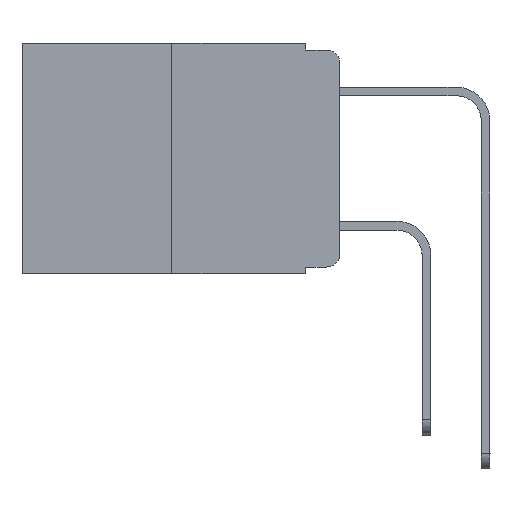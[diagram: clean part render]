
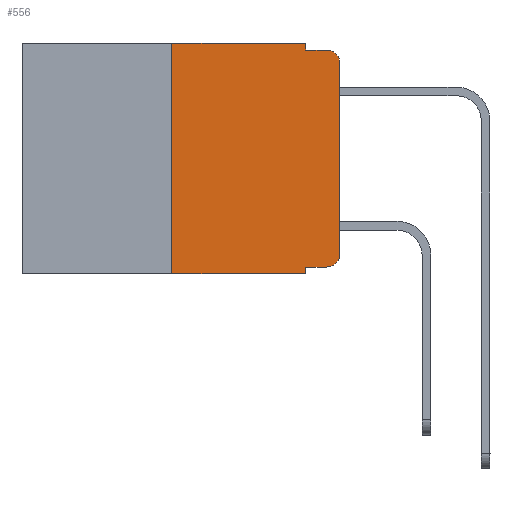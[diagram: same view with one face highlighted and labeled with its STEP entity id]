
A CAD part, left-side view. The second image highlights one B-rep face of the part: STEP entity #556.
In plain terms, the highlighted planar face has unit normal (-1, 0, 0).
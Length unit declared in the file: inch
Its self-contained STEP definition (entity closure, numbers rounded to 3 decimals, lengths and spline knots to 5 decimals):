
#143 = VERTEX_POINT ( 'NONE', #16072 ) ;
#154 = CARTESIAN_POINT ( 'NONE',  ( 0., 0.051, 0. ) ) ;
#478 = EDGE_CURVE ( 'NONE', #11710, #15824, #767, .T. ) ;
#556 = ADVANCED_FACE ( 'NONE', ( #12794 ), #1880, .F. ) ;
#623 = CIRCLE ( 'NONE', #14624, 0.02 ) ;
#665 = AXIS2_PLACEMENT_3D ( 'NONE', #14664, #6798, #13257 ) ;
#767 = LINE ( 'NONE', #4546, #13063 ) ;
#1188 = CARTESIAN_POINT ( 'NONE',  ( 0., 0.051, 0. ) ) ;
#1325 = CARTESIAN_POINT ( 'NONE',  ( 0., 0.051, 0. ) ) ;
#1472 = VERTEX_POINT ( 'NONE', #18660 ) ;
#1818 = DIRECTION ( 'NONE',  ( -1., 0., 0. ) ) ;
#1880 = PLANE ( 'NONE',  #665 ) ;
#1898 = LINE ( 'NONE', #9536, #5864 ) ;
#2449 = DIRECTION ( 'NONE',  ( 0., -1., 0. ) ) ;
#2871 = CIRCLE ( 'NONE', #21621, 0.02 ) ;
#2961 = DIRECTION ( 'NONE',  ( 0., 0., -1. ) ) ;
#3137 = LINE ( 'NONE', #16620, #20459 ) ;
#3693 = DIRECTION ( 'NONE',  ( 0., 0., -1. ) ) ;
#4546 = CARTESIAN_POINT ( 'NONE',  ( 0., 0.473, -0.343 ) ) ;
#5769 = EDGE_CURVE ( 'NONE', #15085, #16753, #2871, .T. ) ;
#5864 = VECTOR ( 'NONE', #17121, 39.37008 ) ;
#6246 = CARTESIAN_POINT ( 'NONE',  ( 0., 0., 0. ) ) ;
#6311 = DIRECTION ( 'NONE',  ( 0., 0., -1. ) ) ;
#6565 = ORIENTED_EDGE ( 'NONE', *, *, #21490, .F. ) ;
#6643 = LINE ( 'NONE', #21256, #14645 ) ;
#6798 = DIRECTION ( 'NONE',  ( 1., 0., 0. ) ) ;
#6861 = LINE ( 'NONE', #1325, #10300 ) ;
#6906 = DIRECTION ( 'NONE',  ( 0., 0., 1. ) ) ;
#6994 = VERTEX_POINT ( 'NONE', #1188 ) ;
#7233 = ORIENTED_EDGE ( 'NONE', *, *, #13101, .T. ) ;
#8119 = LINE ( 'NONE', #6246, #11489 ) ;
#8181 = DIRECTION ( 'NONE',  ( 0., -1., 0. ) ) ;
#9536 = CARTESIAN_POINT ( 'NONE',  ( 0., 0.051, -0.333 ) ) ;
#9826 = CARTESIAN_POINT ( 'NONE',  ( 0., 0., -0.03 ) ) ;
#10131 = DIRECTION ( 'NONE',  ( 0., 0., 1. ) ) ;
#10300 = VECTOR ( 'NONE', #2961, 39.37008 ) ;
#10371 = CARTESIAN_POINT ( 'NONE',  ( 0., 0.02, -0.333 ) ) ;
#10450 = ORIENTED_EDGE ( 'NONE', *, *, #13717, .T. ) ;
#10647 = VECTOR ( 'NONE', #2449, 39.37008 ) ;
#10783 = VERTEX_POINT ( 'NONE', #9826 ) ;
#11489 = VECTOR ( 'NONE', #10131, 39.37008 ) ;
#11710 = VERTEX_POINT ( 'NONE', #14314 ) ;
#12086 = CARTESIAN_POINT ( 'NONE',  ( 0., 0.473, 0. ) ) ;
#12794 = FACE_OUTER_BOUND ( 'NONE', #20873, .T. ) ;
#13063 = VECTOR ( 'NONE', #8181, 39.37008 ) ;
#13101 = EDGE_CURVE ( 'NONE', #1472, #15085, #1898, .T. ) ;
#13153 = DIRECTION ( 'NONE',  ( 0., 0., -1. ) ) ;
#13257 = DIRECTION ( 'NONE',  ( 0., 0., -1. ) ) ;
#13717 = EDGE_CURVE ( 'NONE', #16753, #10783, #8119, .T. ) ;
#13825 = EDGE_CURVE ( 'NONE', #1472, #15824, #6861, .T. ) ;
#14314 = CARTESIAN_POINT ( 'NONE',  ( 0., 0.25, -0.343 ) ) ;
#14583 = EDGE_CURVE ( 'NONE', #6994, #18304, #21531, .T. ) ;
#14624 = AXIS2_PLACEMENT_3D ( 'NONE', #15125, #22879, #13153 ) ;
#14645 = VECTOR ( 'NONE', #15619, 39.37008 ) ;
#14664 = CARTESIAN_POINT ( 'NONE',  ( 0., 0.473, 0. ) ) ;
#14692 = ORIENTED_EDGE ( 'NONE', *, *, #14583, .F. ) ;
#15085 = VERTEX_POINT ( 'NONE', #10371 ) ;
#15125 = CARTESIAN_POINT ( 'NONE',  ( 0., 0.02, -0.03 ) ) ;
#15619 = DIRECTION ( 'NONE',  ( 0., -1., 0. ) ) ;
#15824 = VERTEX_POINT ( 'NONE', #17158 ) ;
#16072 = CARTESIAN_POINT ( 'NONE',  ( 0., 0.02, -0.01 ) ) ;
#16604 = CARTESIAN_POINT ( 'NONE',  ( 0., 0.25, 0. ) ) ;
#16620 = CARTESIAN_POINT ( 'NONE',  ( 0., 0.25, 0. ) ) ;
#16753 = VERTEX_POINT ( 'NONE', #16970 ) ;
#16970 = CARTESIAN_POINT ( 'NONE',  ( 0., 0., -0.313 ) ) ;
#17121 = DIRECTION ( 'NONE',  ( 0., -1., 0. ) ) ;
#17158 = CARTESIAN_POINT ( 'NONE',  ( 0., 0.051, -0.343 ) ) ;
#17756 = EDGE_CURVE ( 'NONE', #11710, #21812, #3137, .T. ) ;
#17838 = VECTOR ( 'NONE', #6311, 39.37008 ) ;
#17901 = LINE ( 'NONE', #12086, #10647 ) ;
#18304 = VERTEX_POINT ( 'NONE', #22839 ) ;
#18660 = CARTESIAN_POINT ( 'NONE',  ( 0., 0.051, -0.333 ) ) ;
#18782 = CARTESIAN_POINT ( 'NONE',  ( 0., 0.02, -0.313 ) ) ;
#18806 = ORIENTED_EDGE ( 'NONE', *, *, #17756, .F. ) ;
#19644 = ORIENTED_EDGE ( 'NONE', *, *, #21778, .F. ) ;
#20091 = ORIENTED_EDGE ( 'NONE', *, *, #5769, .T. ) ;
#20459 = VECTOR ( 'NONE', #6906, 39.37008 ) ;
#20873 = EDGE_LOOP ( 'NONE', ( #10450, #23316, #19644, #14692, #6565, #18806, #21449, #24305, #7233, #20091 ) ) ;
#21256 = CARTESIAN_POINT ( 'NONE',  ( 0., 0.051, -0.01 ) ) ;
#21449 = ORIENTED_EDGE ( 'NONE', *, *, #478, .T. ) ;
#21490 = EDGE_CURVE ( 'NONE', #21812, #6994, #17901, .T. ) ;
#21531 = LINE ( 'NONE', #154, #17838 ) ;
#21565 = EDGE_CURVE ( 'NONE', #10783, #143, #623, .T. ) ;
#21621 = AXIS2_PLACEMENT_3D ( 'NONE', #18782, #1818, #3693 ) ;
#21778 = EDGE_CURVE ( 'NONE', #18304, #143, #6643, .T. ) ;
#21812 = VERTEX_POINT ( 'NONE', #16604 ) ;
#22839 = CARTESIAN_POINT ( 'NONE',  ( 0., 0.051, -0.01 ) ) ;
#22879 = DIRECTION ( 'NONE',  ( -1., 0., 0. ) ) ;
#23316 = ORIENTED_EDGE ( 'NONE', *, *, #21565, .T. ) ;
#24305 = ORIENTED_EDGE ( 'NONE', *, *, #13825, .F. ) ;
